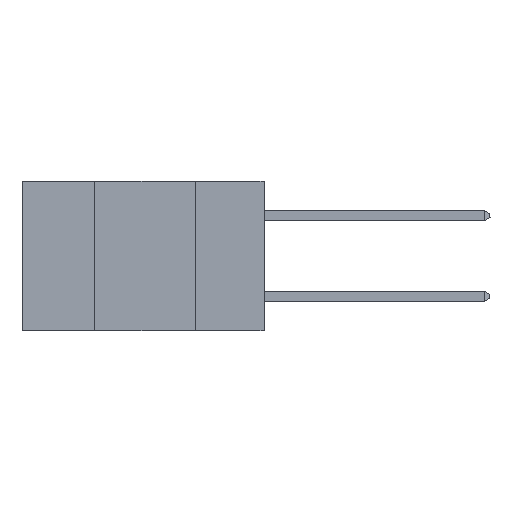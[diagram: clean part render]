
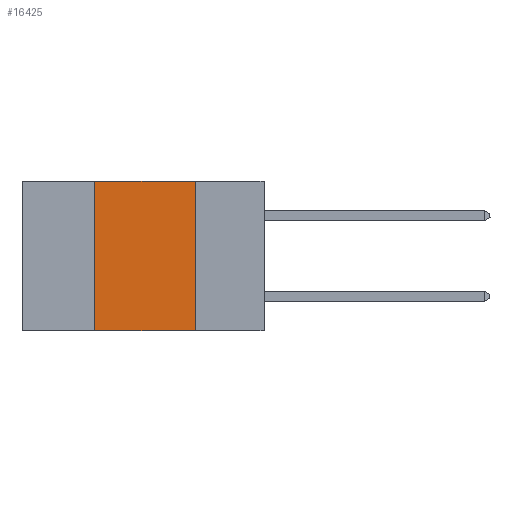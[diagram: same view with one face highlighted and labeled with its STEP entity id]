
A CAD part, left-side view. The second image highlights one B-rep face of the part: STEP entity #16425.
In plain terms, the highlighted planar face has unit normal (-1, 0, 0).
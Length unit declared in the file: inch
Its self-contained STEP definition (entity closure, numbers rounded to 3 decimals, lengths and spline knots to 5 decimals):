
#299 = VECTOR ( 'NONE', #5263, 39.37008 ) ;
#1414 = CARTESIAN_POINT ( 'NONE',  ( 0., 0.6, -0.37 ) ) ;
#2020 = CARTESIAN_POINT ( 'NONE',  ( 0., 0.42, 0. ) ) ;
#3615 = CARTESIAN_POINT ( 'NONE',  ( 0., 0.17, 0. ) ) ;
#3668 = LINE ( 'NONE', #22717, #22524 ) ;
#5263 = DIRECTION ( 'NONE',  ( 0., -1., 0. ) ) ;
#5404 = FACE_OUTER_BOUND ( 'NONE', #31890, .T. ) ;
#7204 = AXIS2_PLACEMENT_3D ( 'NONE', #23939, #13706, #29226 ) ;
#11028 = VECTOR ( 'NONE', #26982, 39.37008 ) ;
#11581 = EDGE_CURVE ( 'NONE', #29071, #19198, #18775, .T. ) ;
#12525 = EDGE_CURVE ( 'NONE', #23784, #15966, #13836, .T. ) ;
#13706 = DIRECTION ( 'NONE',  ( 1., 0., 0. ) ) ;
#13836 = LINE ( 'NONE', #1414, #11028 ) ;
#14917 = ORIENTED_EDGE ( 'NONE', *, *, #20126, .F. ) ;
#14939 = DIRECTION ( 'NONE',  ( 0., 0., -1. ) ) ;
#15664 = CARTESIAN_POINT ( 'NONE',  ( 0., 0.17, -0.37 ) ) ;
#15966 = VERTEX_POINT ( 'NONE', #15664 ) ;
#16425 = ADVANCED_FACE ( 'NONE', ( #5404 ), #26625, .F. ) ;
#17519 = CARTESIAN_POINT ( 'NONE',  ( 0., 0.17, 0. ) ) ;
#18025 = DIRECTION ( 'NONE',  ( 0., 0., 1. ) ) ;
#18655 = ORIENTED_EDGE ( 'NONE', *, *, #12525, .T. ) ;
#18775 = LINE ( 'NONE', #25679, #299 ) ;
#19198 = VERTEX_POINT ( 'NONE', #3615 ) ;
#20126 = EDGE_CURVE ( 'NONE', #23784, #29071, #3668, .T. ) ;
#20827 = LINE ( 'NONE', #17519, #26052 ) ;
#22524 = VECTOR ( 'NONE', #18025, 39.37008 ) ;
#22717 = CARTESIAN_POINT ( 'NONE',  ( 0., 0.42, 0. ) ) ;
#23784 = VERTEX_POINT ( 'NONE', #30357 ) ;
#23939 = CARTESIAN_POINT ( 'NONE',  ( 0., 0.6, 0. ) ) ;
#25679 = CARTESIAN_POINT ( 'NONE',  ( 0., 0.6, 0. ) ) ;
#26052 = VECTOR ( 'NONE', #14939, 39.37008 ) ;
#26625 = PLANE ( 'NONE',  #7204 ) ;
#26982 = DIRECTION ( 'NONE',  ( 0., -1., 0. ) ) ;
#27568 = ORIENTED_EDGE ( 'NONE', *, *, #28870, .F. ) ;
#28870 = EDGE_CURVE ( 'NONE', #19198, #15966, #20827, .T. ) ;
#29071 = VERTEX_POINT ( 'NONE', #2020 ) ;
#29226 = DIRECTION ( 'NONE',  ( 0., 0., -1. ) ) ;
#29914 = ORIENTED_EDGE ( 'NONE', *, *, #11581, .F. ) ;
#30357 = CARTESIAN_POINT ( 'NONE',  ( 0., 0.42, -0.37 ) ) ;
#31890 = EDGE_LOOP ( 'NONE', ( #27568, #29914, #14917, #18655 ) ) ;
